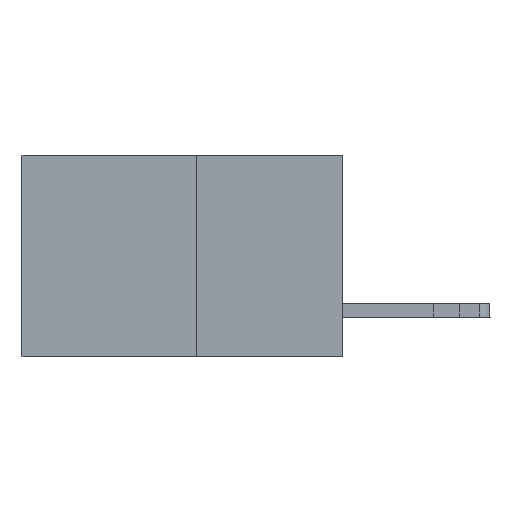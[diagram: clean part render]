
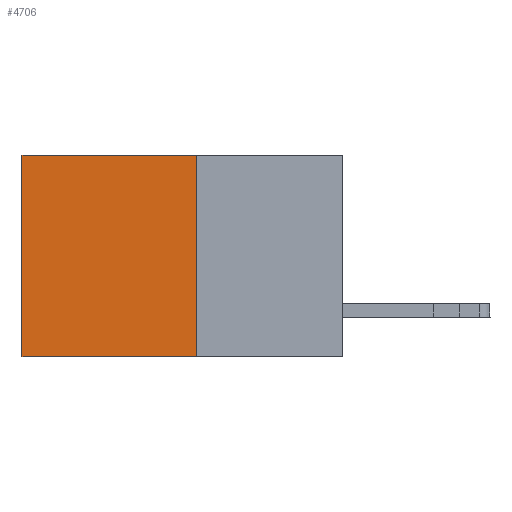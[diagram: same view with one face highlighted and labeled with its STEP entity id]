
A CAD part, left-side view. The second image highlights one B-rep face of the part: STEP entity #4706.
In plain terms, the highlighted planar face has unit normal (-1, 0, 0).
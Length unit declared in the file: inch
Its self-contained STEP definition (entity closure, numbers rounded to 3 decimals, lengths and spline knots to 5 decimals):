
#366 = ORIENTED_EDGE ( 'NONE', *, *, #4746, .T. ) ;
#1029 = VERTEX_POINT ( 'NONE', #6669 ) ;
#1272 = VECTOR ( 'NONE', #5987, 39.37008 ) ;
#1998 = CARTESIAN_POINT ( 'NONE',  ( 0.277, 0.59, -0.37 ) ) ;
#2679 = CARTESIAN_POINT ( 'NONE',  ( 0.277, 0.59, -0.37 ) ) ;
#2736 = DIRECTION ( 'NONE',  ( 0., 0., -1. ) ) ;
#2855 = VECTOR ( 'NONE', #14107, 39.37008 ) ;
#3047 = EDGE_LOOP ( 'NONE', ( #366, #13119, #12901, #8297 ) ) ;
#3061 = VERTEX_POINT ( 'NONE', #2679 ) ;
#3547 = CARTESIAN_POINT ( 'NONE',  ( 0.277, 0.27, -0.37 ) ) ;
#3771 = CARTESIAN_POINT ( 'NONE',  ( 0.277, 0.59, 0. ) ) ;
#3834 = PLANE ( 'NONE',  #6268 ) ;
#4706 = ADVANCED_FACE ( 'NONE', ( #9370 ), #3834, .F. ) ;
#4746 = EDGE_CURVE ( 'NONE', #10100, #3061, #10677, .T. ) ;
#5987 = DIRECTION ( 'NONE',  ( 0., 0., -1. ) ) ;
#6121 = EDGE_CURVE ( 'NONE', #1029, #10100, #6476, .T. ) ;
#6268 = AXIS2_PLACEMENT_3D ( 'NONE', #12728, #6790, #2736 ) ;
#6476 = LINE ( 'NONE', #9664, #2855 ) ;
#6669 = CARTESIAN_POINT ( 'NONE',  ( 0.277, 0.27, 0. ) ) ;
#6790 = DIRECTION ( 'NONE',  ( 1., 0., 0. ) ) ;
#7776 = EDGE_CURVE ( 'NONE', #1029, #8682, #12755, .T. ) ;
#7996 = DIRECTION ( 'NONE',  ( 0., 1., 0. ) ) ;
#8297 = ORIENTED_EDGE ( 'NONE', *, *, #6121, .T. ) ;
#8577 = DIRECTION ( 'NONE',  ( 0., 0., -1. ) ) ;
#8682 = VERTEX_POINT ( 'NONE', #10303 ) ;
#9370 = FACE_OUTER_BOUND ( 'NONE', #3047, .T. ) ;
#9664 = CARTESIAN_POINT ( 'NONE',  ( 0.277, 0.27, 0. ) ) ;
#10100 = VERTEX_POINT ( 'NONE', #3771 ) ;
#10303 = CARTESIAN_POINT ( 'NONE',  ( 0.277, 0.27, -0.37 ) ) ;
#10677 = LINE ( 'NONE', #1998, #13246 ) ;
#11866 = CARTESIAN_POINT ( 'NONE',  ( 0.277, 0.27, -0.37 ) ) ;
#12728 = CARTESIAN_POINT ( 'NONE',  ( 0.277, 0.27, -0.37 ) ) ;
#12755 = LINE ( 'NONE', #11866, #1272 ) ;
#12901 = ORIENTED_EDGE ( 'NONE', *, *, #7776, .F. ) ;
#13119 = ORIENTED_EDGE ( 'NONE', *, *, #13766, .F. ) ;
#13246 = VECTOR ( 'NONE', #8577, 39.37008 ) ;
#13527 = LINE ( 'NONE', #3547, #14374 ) ;
#13766 = EDGE_CURVE ( 'NONE', #8682, #3061, #13527, .T. ) ;
#14107 = DIRECTION ( 'NONE',  ( 0., 1., 0. ) ) ;
#14374 = VECTOR ( 'NONE', #7996, 39.37008 ) ;
